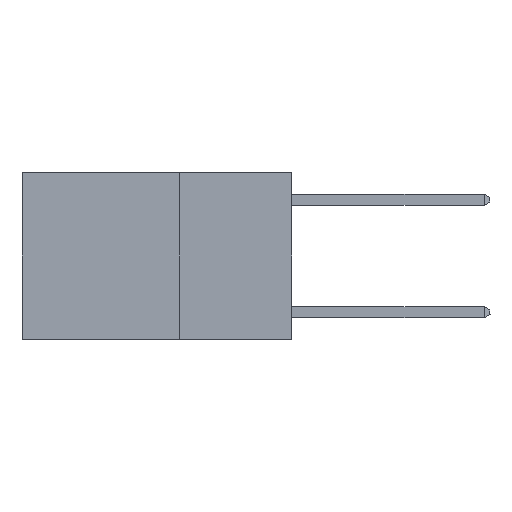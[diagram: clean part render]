
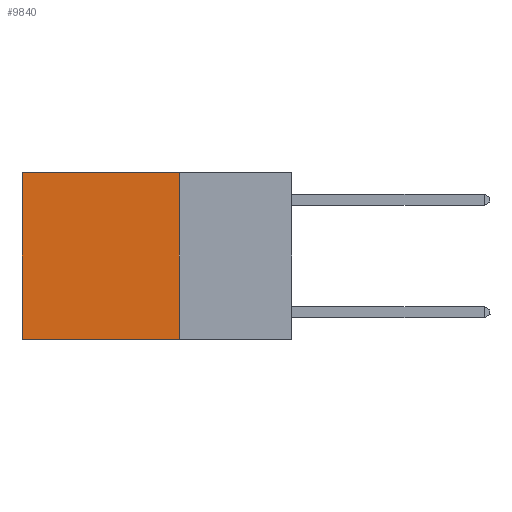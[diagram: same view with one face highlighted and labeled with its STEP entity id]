
A CAD part, left-side view. The second image highlights one B-rep face of the part: STEP entity #9840.
In plain terms, the highlighted planar face has unit normal (-1, 0, 0).
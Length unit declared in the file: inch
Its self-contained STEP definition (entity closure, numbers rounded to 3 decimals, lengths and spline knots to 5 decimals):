
#155 = VERTEX_POINT ( 'NONE', #14245 ) ;
#1168 = EDGE_CURVE ( 'NONE', #13900, #13214, #10332, .T. ) ;
#1190 = EDGE_CURVE ( 'NONE', #5963, #155, #2339, .T. ) ;
#1391 = CARTESIAN_POINT ( 'NONE',  ( 0.2625, 0.25, 0. ) ) ;
#1462 = ORIENTED_EDGE ( 'NONE', *, *, #7389, .T. ) ;
#2114 = PLANE ( 'NONE',  #12482 ) ;
#2339 = LINE ( 'NONE', #14155, #13459 ) ;
#2572 = EDGE_CURVE ( 'NONE', #13214, #155, #3707, .T. ) ;
#2692 = DIRECTION ( 'NONE',  ( 0., 1., 0. ) ) ;
#2741 = VECTOR ( 'NONE', #15365, 39.37008 ) ;
#3402 = DIRECTION ( 'NONE',  ( 1., 0., 0. ) ) ;
#3523 = CARTESIAN_POINT ( 'NONE',  ( 0.2625, 0.6, 0. ) ) ;
#3707 = LINE ( 'NONE', #15489, #14017 ) ;
#4074 = ORIENTED_EDGE ( 'NONE', *, *, #1168, .F. ) ;
#4222 = CARTESIAN_POINT ( 'NONE',  ( 0.2625, 0.25, 0. ) ) ;
#4537 = VECTOR ( 'NONE', #2692, 39.37008 ) ;
#4610 = EDGE_LOOP ( 'NONE', ( #6729, #8587, #4074, #1462 ) ) ;
#4636 = CARTESIAN_POINT ( 'NONE',  ( 0.2625, 0.25, 0. ) ) ;
#4754 = DIRECTION ( 'NONE',  ( 0., 0., -1. ) ) ;
#5836 = CARTESIAN_POINT ( 'NONE',  ( 0.2625, 0.25, -0.37 ) ) ;
#5963 = VERTEX_POINT ( 'NONE', #3523 ) ;
#6729 = ORIENTED_EDGE ( 'NONE', *, *, #1190, .T. ) ;
#7389 = EDGE_CURVE ( 'NONE', #13900, #5963, #7714, .T. ) ;
#7714 = LINE ( 'NONE', #1391, #4537 ) ;
#8587 = ORIENTED_EDGE ( 'NONE', *, *, #2572, .F. ) ;
#9343 = FACE_OUTER_BOUND ( 'NONE', #4610, .T. ) ;
#9840 = ADVANCED_FACE ( 'NONE', ( #9343 ), #2114, .F. ) ;
#10145 = CARTESIAN_POINT ( 'NONE',  ( 0.2625, 0.25, 0. ) ) ;
#10332 = LINE ( 'NONE', #4636, #2741 ) ;
#12482 = AXIS2_PLACEMENT_3D ( 'NONE', #10145, #3402, #12873 ) ;
#12873 = DIRECTION ( 'NONE',  ( 0., 0., -1. ) ) ;
#12959 = DIRECTION ( 'NONE',  ( 0., 1., 0. ) ) ;
#13214 = VERTEX_POINT ( 'NONE', #5836 ) ;
#13459 = VECTOR ( 'NONE', #4754, 39.37008 ) ;
#13900 = VERTEX_POINT ( 'NONE', #4222 ) ;
#14017 = VECTOR ( 'NONE', #12959, 39.37008 ) ;
#14155 = CARTESIAN_POINT ( 'NONE',  ( 0.2625, 0.6, 0. ) ) ;
#14245 = CARTESIAN_POINT ( 'NONE',  ( 0.2625, 0.6, -0.37 ) ) ;
#15365 = DIRECTION ( 'NONE',  ( 0., 0., -1. ) ) ;
#15489 = CARTESIAN_POINT ( 'NONE',  ( 0.2625, 0.25, -0.37 ) ) ;
